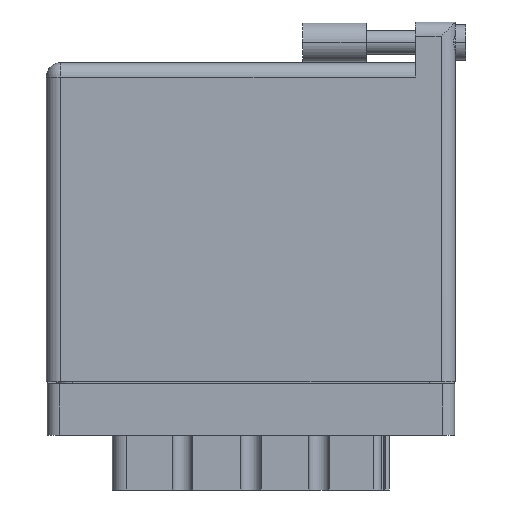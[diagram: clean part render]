
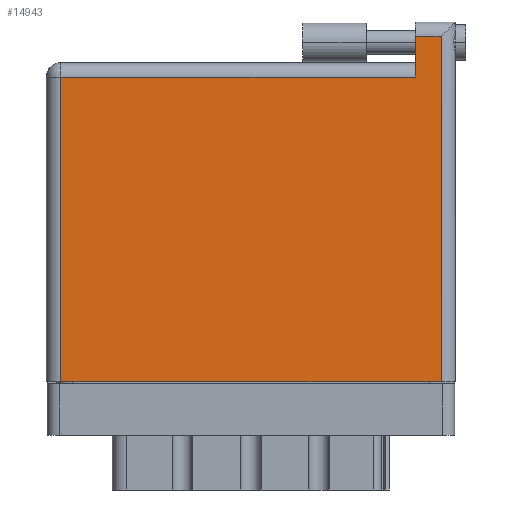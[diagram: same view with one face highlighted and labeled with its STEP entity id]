
A CAD part, front view. The second image highlights one B-rep face of the part: STEP entity #14943.
In plain terms, the highlighted face is planar.
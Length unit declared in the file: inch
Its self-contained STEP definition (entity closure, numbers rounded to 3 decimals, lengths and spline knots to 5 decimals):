
#880 = EDGE_CURVE ( 'NONE', #21572, #1292, #40067, .T. ) ;
#1292 = VERTEX_POINT ( 'NONE', #13901 ) ;
#2089 = DIRECTION ( 'NONE',  ( 0., -1., 0. ) ) ;
#2931 = VECTOR ( 'NONE', #33144, 39.37008 ) ;
#7292 = EDGE_CURVE ( 'NONE', #8900, #40816, #41010, .T. ) ;
#7413 = ORIENTED_EDGE ( 'NONE', *, *, #7292, .T. ) ;
#8900 = VERTEX_POINT ( 'NONE', #14872 ) ;
#9059 = VECTOR ( 'NONE', #2089, 39.37008 ) ;
#9208 = DIRECTION ( 'NONE',  ( 0., 1., 0. ) ) ;
#9885 = CARTESIAN_POINT ( 'NONE',  ( 0., 1.496, 0. ) ) ;
#11922 = LINE ( 'NONE', #9885, #32301 ) ;
#12719 = CARTESIAN_POINT ( 'NONE',  ( 1.811, 1.696, 0. ) ) ;
#12914 = DIRECTION ( 'NONE',  ( -1., 0., 0. ) ) ;
#13901 = CARTESIAN_POINT ( 'NONE',  ( 1.938, 0., 0. ) ) ;
#14539 = FACE_OUTER_BOUND ( 'NONE', #18807, .T. ) ;
#14872 = CARTESIAN_POINT ( 'NONE',  ( 1.938, 1.696, 0. ) ) ;
#14943 = ADVANCED_FACE ( 'NONE', ( #14539 ), #20473, .F. ) ;
#15352 = CARTESIAN_POINT ( 'NONE',  ( 1.938, 1.766, 0. ) ) ;
#15449 = ORIENTED_EDGE ( 'NONE', *, *, #34323, .T. ) ;
#16164 = DIRECTION ( 'NONE',  ( -1., 0., 0. ) ) ;
#17252 = DIRECTION ( 'NONE',  ( 1., 0., 0. ) ) ;
#17419 = CARTESIAN_POINT ( 'NONE',  ( 0., 1.566, 0. ) ) ;
#18807 = EDGE_LOOP ( 'NONE', ( #36302, #36568, #7413, #15449, #21880, #22417 ) ) ;
#19539 = LINE ( 'NONE', #35818, #9059 ) ;
#19813 = LINE ( 'NONE', #29502, #2931 ) ;
#20473 = PLANE ( 'NONE',  #34573 ) ;
#20614 = DIRECTION ( 'NONE',  ( -1., 0., 0. ) ) ;
#20819 = CARTESIAN_POINT ( 'NONE',  ( 1.811, 1.496, 0. ) ) ;
#21572 = VERTEX_POINT ( 'NONE', #35460 ) ;
#21880 = ORIENTED_EDGE ( 'NONE', *, *, #26091, .T. ) ;
#22417 = ORIENTED_EDGE ( 'NONE', *, *, #31891, .T. ) ;
#23738 = LINE ( 'NONE', #15352, #41164 ) ;
#26091 = EDGE_CURVE ( 'NONE', #36058, #38225, #11922, .T. ) ;
#26905 = CARTESIAN_POINT ( 'NONE',  ( 0.07, 1.496, 0. ) ) ;
#28095 = VECTOR ( 'NONE', #12914, 39.37008 ) ;
#28116 = VECTOR ( 'NONE', #17252, 39.37008 ) ;
#29502 = CARTESIAN_POINT ( 'NONE',  ( 1.811, 1.766, 0. ) ) ;
#31891 = EDGE_CURVE ( 'NONE', #38225, #21572, #19539, .T. ) ;
#32301 = VECTOR ( 'NONE', #16164, 39.37008 ) ;
#33144 = DIRECTION ( 'NONE',  ( 0., -1., 0. ) ) ;
#34323 = EDGE_CURVE ( 'NONE', #40816, #36058, #19813, .T. ) ;
#34573 = AXIS2_PLACEMENT_3D ( 'NONE', #17419, #39039, #20614 ) ;
#34925 = EDGE_CURVE ( 'NONE', #1292, #8900, #23738, .T. ) ;
#35118 = CARTESIAN_POINT ( 'NONE',  ( 0., 1.696, 0. ) ) ;
#35460 = CARTESIAN_POINT ( 'NONE',  ( 0.07, 0., 0. ) ) ;
#35818 = CARTESIAN_POINT ( 'NONE',  ( 0.07, 0., 0. ) ) ;
#36058 = VERTEX_POINT ( 'NONE', #20819 ) ;
#36302 = ORIENTED_EDGE ( 'NONE', *, *, #880, .T. ) ;
#36568 = ORIENTED_EDGE ( 'NONE', *, *, #34925, .T. ) ;
#36816 = CARTESIAN_POINT ( 'NONE',  ( 0., 0., 0. ) ) ;
#38225 = VERTEX_POINT ( 'NONE', #26905 ) ;
#39039 = DIRECTION ( 'NONE',  ( 0., 0., -1. ) ) ;
#40067 = LINE ( 'NONE', #36816, #28116 ) ;
#40816 = VERTEX_POINT ( 'NONE', #12719 ) ;
#41010 = LINE ( 'NONE', #35118, #28095 ) ;
#41164 = VECTOR ( 'NONE', #9208, 39.37008 ) ;
